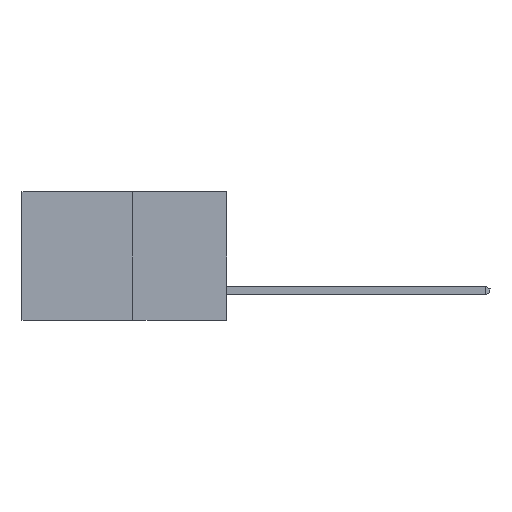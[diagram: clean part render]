
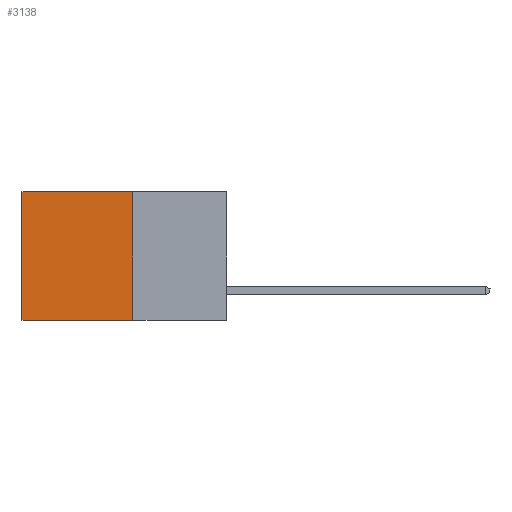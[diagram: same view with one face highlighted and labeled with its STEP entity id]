
A CAD part, left-side view. The second image highlights one B-rep face of the part: STEP entity #3138.
In plain terms, the highlighted planar face has unit normal (-1, 0, 0).
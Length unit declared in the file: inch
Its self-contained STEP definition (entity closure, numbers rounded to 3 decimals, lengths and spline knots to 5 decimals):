
#83 = ORIENTED_EDGE ( 'NONE', *, *, #4365, .F. ) ;
#1215 = ORIENTED_EDGE ( 'NONE', *, *, #4577, .T. ) ;
#1561 = VECTOR ( 'NONE', #3568, 39.37008 ) ;
#2721 = VECTOR ( 'NONE', #2888, 39.37008 ) ;
#2888 = DIRECTION ( 'NONE',  ( 0., 0., -1. ) ) ;
#3037 = FACE_OUTER_BOUND ( 'NONE', #6945, .T. ) ;
#3138 = ADVANCED_FACE ( 'NONE', ( #3037 ), #7710, .F. ) ;
#3343 = DIRECTION ( 'NONE',  ( 0., 1., 0. ) ) ;
#3568 = DIRECTION ( 'NONE',  ( 0., 0., -1. ) ) ;
#3851 = VERTEX_POINT ( 'NONE', #8163 ) ;
#4365 = EDGE_CURVE ( 'NONE', #8383, #3851, #9655, .T. ) ;
#4459 = ORIENTED_EDGE ( 'NONE', *, *, #11915, .F. ) ;
#4577 = EDGE_CURVE ( 'NONE', #10499, #3851, #5551, .T. ) ;
#4862 = VECTOR ( 'NONE', #9212, 39.37008 ) ;
#5404 = ORIENTED_EDGE ( 'NONE', *, *, #11759, .T. ) ;
#5551 = LINE ( 'NONE', #6685, #2721 ) ;
#5592 = LINE ( 'NONE', #10667, #10124 ) ;
#6216 = VERTEX_POINT ( 'NONE', #10057 ) ;
#6685 = CARTESIAN_POINT ( 'NONE',  ( 0.277, 0.59, -0.37 ) ) ;
#6945 = EDGE_LOOP ( 'NONE', ( #1215, #83, #4459, #5404 ) ) ;
#7710 = PLANE ( 'NONE',  #10843 ) ;
#7790 = DIRECTION ( 'NONE',  ( 0., 0., -1. ) ) ;
#7813 = CARTESIAN_POINT ( 'NONE',  ( 0.277, 0.27, -0.37 ) ) ;
#7831 = CARTESIAN_POINT ( 'NONE',  ( 0.277, 0.27, -0.37 ) ) ;
#7918 = CARTESIAN_POINT ( 'NONE',  ( 0.277, 0.27, -0.37 ) ) ;
#8163 = CARTESIAN_POINT ( 'NONE',  ( 0.277, 0.59, -0.37 ) ) ;
#8180 = CARTESIAN_POINT ( 'NONE',  ( 0.277, 0.27, -0.37 ) ) ;
#8383 = VERTEX_POINT ( 'NONE', #7831 ) ;
#9212 = DIRECTION ( 'NONE',  ( 0., 1., 0. ) ) ;
#9274 = LINE ( 'NONE', #8180, #1561 ) ;
#9655 = LINE ( 'NONE', #7918, #4862 ) ;
#10057 = CARTESIAN_POINT ( 'NONE',  ( 0.277, 0.27, 0. ) ) ;
#10074 = CARTESIAN_POINT ( 'NONE',  ( 0.277, 0.59, 0. ) ) ;
#10124 = VECTOR ( 'NONE', #3343, 39.37008 ) ;
#10499 = VERTEX_POINT ( 'NONE', #10074 ) ;
#10667 = CARTESIAN_POINT ( 'NONE',  ( 0.277, 0.27, 0. ) ) ;
#10843 = AXIS2_PLACEMENT_3D ( 'NONE', #7813, #11648, #7790 ) ;
#11648 = DIRECTION ( 'NONE',  ( 1., 0., 0. ) ) ;
#11759 = EDGE_CURVE ( 'NONE', #6216, #10499, #5592, .T. ) ;
#11915 = EDGE_CURVE ( 'NONE', #6216, #8383, #9274, .T. ) ;
